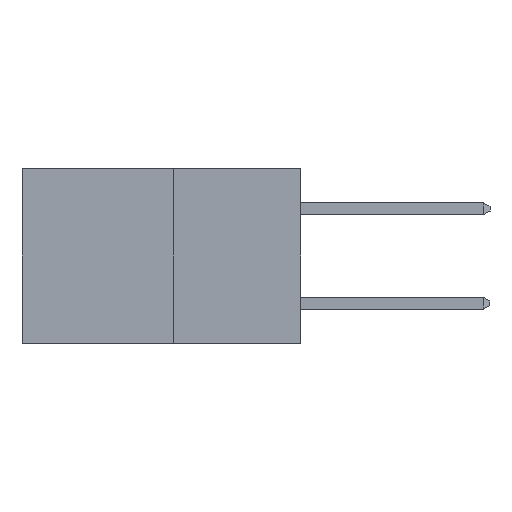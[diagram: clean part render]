
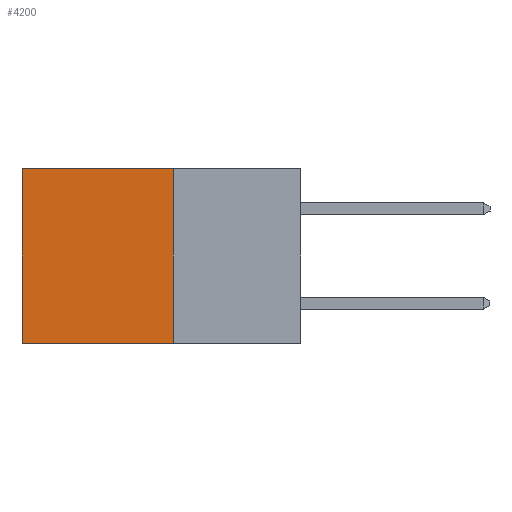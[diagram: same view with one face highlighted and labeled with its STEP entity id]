
A CAD part, left-side view. The second image highlights one B-rep face of the part: STEP entity #4200.
In plain terms, the highlighted planar face has unit normal (-1, 0, 0).
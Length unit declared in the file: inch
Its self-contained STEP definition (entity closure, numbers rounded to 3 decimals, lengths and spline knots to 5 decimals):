
#8 = CARTESIAN_POINT ( 'NONE',  ( 0.277, 0.27, 0. ) ) ;
#41 = DIRECTION ( 'NONE',  ( 0., 1., 0. ) ) ;
#211 = CARTESIAN_POINT ( 'NONE',  ( 0.277, 0.27, -0.37 ) ) ;
#594 = CARTESIAN_POINT ( 'NONE',  ( 0.277, 0.27, -0.37 ) ) ;
#938 = EDGE_CURVE ( 'NONE', #7032, #1235, #6225, .T. ) ;
#1235 = VERTEX_POINT ( 'NONE', #6289 ) ;
#1238 = ORIENTED_EDGE ( 'NONE', *, *, #5127, .F. ) ;
#1288 = VECTOR ( 'NONE', #2448, 39.37008 ) ;
#1679 = VERTEX_POINT ( 'NONE', #6753 ) ;
#1922 = VERTEX_POINT ( 'NONE', #594 ) ;
#2292 = EDGE_CURVE ( 'NONE', #1235, #1679, #3806, .T. ) ;
#2362 = EDGE_CURVE ( 'NONE', #7032, #1922, #3227, .T. ) ;
#2378 = VECTOR ( 'NONE', #41, 39.37008 ) ;
#2448 = DIRECTION ( 'NONE',  ( 0., 1., 0. ) ) ;
#2556 = ORIENTED_EDGE ( 'NONE', *, *, #2362, .F. ) ;
#2589 = FACE_OUTER_BOUND ( 'NONE', #3073, .T. ) ;
#2678 = AXIS2_PLACEMENT_3D ( 'NONE', #7709, #7583, #2841 ) ;
#2841 = DIRECTION ( 'NONE',  ( 0., 0., -1. ) ) ;
#2958 = LINE ( 'NONE', #211, #2378 ) ;
#3073 = EDGE_LOOP ( 'NONE', ( #5698, #1238, #2556, #4096 ) ) ;
#3227 = LINE ( 'NONE', #7859, #4636 ) ;
#3806 = LINE ( 'NONE', #4539, #6119 ) ;
#4096 = ORIENTED_EDGE ( 'NONE', *, *, #938, .T. ) ;
#4200 = ADVANCED_FACE ( 'NONE', ( #2589 ), #6110, .F. ) ;
#4249 = DIRECTION ( 'NONE',  ( 0., 0., -1. ) ) ;
#4539 = CARTESIAN_POINT ( 'NONE',  ( 0.277, 0.59, -0.37 ) ) ;
#4594 = DIRECTION ( 'NONE',  ( 0., 0., -1. ) ) ;
#4636 = VECTOR ( 'NONE', #4249, 39.37008 ) ;
#5127 = EDGE_CURVE ( 'NONE', #1922, #1679, #2958, .T. ) ;
#5698 = ORIENTED_EDGE ( 'NONE', *, *, #2292, .T. ) ;
#6110 = PLANE ( 'NONE',  #2678 ) ;
#6119 = VECTOR ( 'NONE', #4594, 39.37008 ) ;
#6225 = LINE ( 'NONE', #6709, #1288 ) ;
#6289 = CARTESIAN_POINT ( 'NONE',  ( 0.277, 0.59, 0. ) ) ;
#6709 = CARTESIAN_POINT ( 'NONE',  ( 0.277, 0.27, 0. ) ) ;
#6753 = CARTESIAN_POINT ( 'NONE',  ( 0.277, 0.59, -0.37 ) ) ;
#7032 = VERTEX_POINT ( 'NONE', #8 ) ;
#7583 = DIRECTION ( 'NONE',  ( 1., 0., 0. ) ) ;
#7709 = CARTESIAN_POINT ( 'NONE',  ( 0.277, 0.27, -0.37 ) ) ;
#7859 = CARTESIAN_POINT ( 'NONE',  ( 0.277, 0.27, -0.37 ) ) ;
